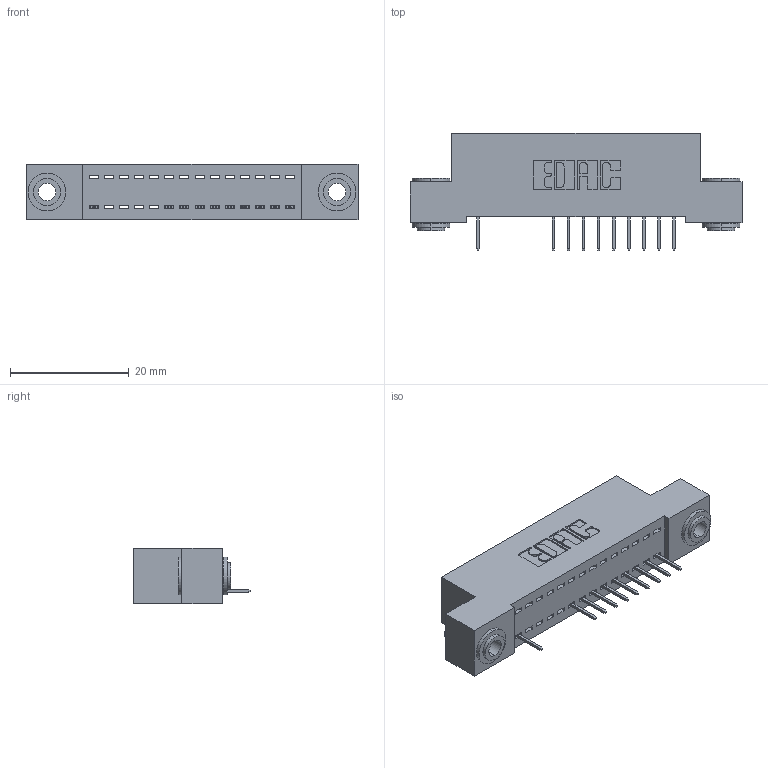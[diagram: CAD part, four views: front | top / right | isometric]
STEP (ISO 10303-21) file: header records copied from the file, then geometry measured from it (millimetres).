
FILE_DESCRIPTION (( 'STEP AP203' ), '1' );
FILE_NAME ('392-014-524-103.STEP', '2018-08-14T23:43:00', ( '' ), ( '' ), 'SwSTEP 2.0', 'SolidWorks 2016', '' );
FILE_SCHEMA (( 'CONFIG_CONTROL_DESIGN' ));
Length unit declared in the file: inch
Products named in the file (4): 392-014-524-103; 342 Part_.156 TH; 345-292-001_345-293-124; 342-250-002_345-250-002-102
Assembly tree (13 placements, depth 2):
  392-014-524-103
    342 Part_.156 TH
    345-292-001_345-293-124  x10
    342-250-002_345-250-002-102  x2
Bounding box: 55.88 x 19.69 x 9.4 mm (x, y, z)
Volume: 4734 mm3; surface area: 6295.3 mm2
Topology: 13 solids, 13 shells, 816 faces, 2343 edges, 1518 vertices
Faces by surface type: plane 604, cylinder 204, cone 8
Entity records: 12644 total; most frequent: CARTESIAN_POINT 2179, ORIENTED_EDGE 2126, DIRECTION 1925, EDGE_CURVE 1063, LINE 915, VECTOR 915, VERTEX_POINT 702, AXIS2_PLACEMENT_3D 505
